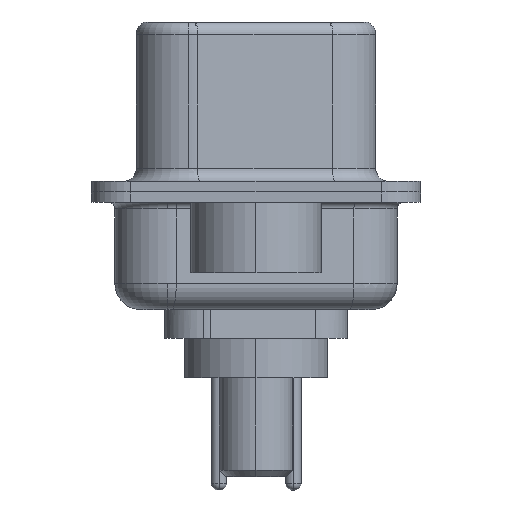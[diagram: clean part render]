
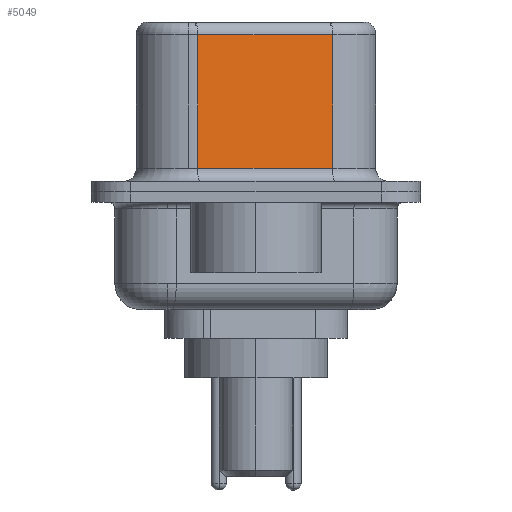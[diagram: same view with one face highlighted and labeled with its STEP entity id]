
A CAD part, left-side view. The second image highlights one B-rep face of the part: STEP entity #5049.
In plain terms, the highlighted planar face has unit normal (-0.985, -0.174, 0).
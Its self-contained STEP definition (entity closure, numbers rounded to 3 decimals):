
#18 = CARTESIAN_POINT ( 'NONE',  ( 3.67, 2.233, 0.9 ) ) ;
#423 = ORIENTED_EDGE ( 'NONE', *, *, #17181, .T. ) ;
#1041 = EDGE_CURVE ( 'NONE', #16443, #9297, #13891, .T. ) ;
#1736 = CARTESIAN_POINT ( 'NONE',  ( 4.58, -2.927, 6.52 ) ) ;
#2870 = PLANE ( 'NONE',  #18915 ) ;
#5049 = ADVANCED_FACE ( 'NONE', ( #21084 ), #2870, .F. ) ;
#5467 = EDGE_CURVE ( 'NONE', #9297, #15932, #8486, .T. ) ;
#6228 = VECTOR ( 'NONE', #21644, 1000. ) ;
#6799 = LINE ( 'NONE', #7184, #16625 ) ;
#7126 = DIRECTION ( 'NONE',  ( -0.174, 0.985, 0. ) ) ;
#7183 = DIRECTION ( 'NONE',  ( 0.985, 0.174, 0. ) ) ;
#7184 = CARTESIAN_POINT ( 'NONE',  ( 4.58, -2.927, 6.52 ) ) ;
#7530 = CARTESIAN_POINT ( 'NONE',  ( 3.67, 2.233, 6.02 ) ) ;
#7801 = ORIENTED_EDGE ( 'NONE', *, *, #18253, .F. ) ;
#7918 = CARTESIAN_POINT ( 'NONE',  ( 4.58, -2.927, 6.02 ) ) ;
#8486 = LINE ( 'NONE', #24946, #23528 ) ;
#9292 = VECTOR ( 'NONE', #20146, 1000. ) ;
#9297 = VERTEX_POINT ( 'NONE', #18 ) ;
#13891 = LINE ( 'NONE', #21856, #9292 ) ;
#15419 = CARTESIAN_POINT ( 'NONE',  ( 4.58, -2.927, 0.9 ) ) ;
#15932 = VERTEX_POINT ( 'NONE', #15419 ) ;
#16255 = CARTESIAN_POINT ( 'NONE',  ( 4.58, -2.927, 6.02 ) ) ;
#16443 = VERTEX_POINT ( 'NONE', #7530 ) ;
#16625 = VECTOR ( 'NONE', #20877, 1000. ) ;
#16739 = VERTEX_POINT ( 'NONE', #16255 ) ;
#17181 = EDGE_CURVE ( 'NONE', #16739, #16443, #21258, .T. ) ;
#18253 = EDGE_CURVE ( 'NONE', #16739, #15932, #6799, .T. ) ;
#18915 = AXIS2_PLACEMENT_3D ( 'NONE', #1736, #7183, #7126 ) ;
#20146 = DIRECTION ( 'NONE',  ( 0., 0., -1. ) ) ;
#20877 = DIRECTION ( 'NONE',  ( 0., 0., -1. ) ) ;
#20886 = DIRECTION ( 'NONE',  ( 0.174, -0.985, 0. ) ) ;
#21084 = FACE_OUTER_BOUND ( 'NONE', #23909, .T. ) ;
#21258 = LINE ( 'NONE', #7918, #6228 ) ;
#21644 = DIRECTION ( 'NONE',  ( -0.174, 0.985, 0. ) ) ;
#21856 = CARTESIAN_POINT ( 'NONE',  ( 3.67, 2.233, 6.52 ) ) ;
#22648 = ORIENTED_EDGE ( 'NONE', *, *, #1041, .T. ) ;
#23528 = VECTOR ( 'NONE', #20886, 1000. ) ;
#23909 = EDGE_LOOP ( 'NONE', ( #7801, #423, #22648, #25150 ) ) ;
#24946 = CARTESIAN_POINT ( 'NONE',  ( 4.58, -2.927, 0.9 ) ) ;
#25150 = ORIENTED_EDGE ( 'NONE', *, *, #5467, .T. ) ;
